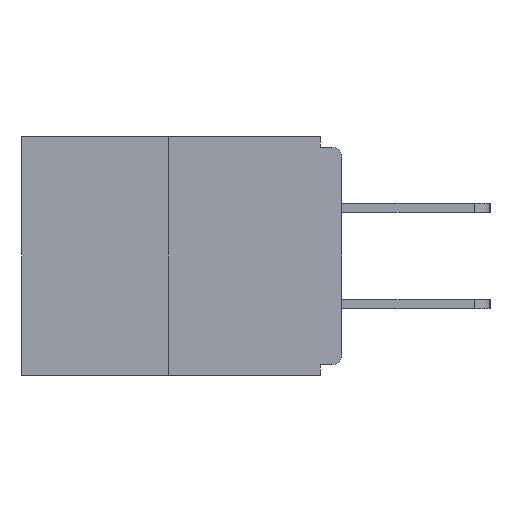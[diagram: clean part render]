
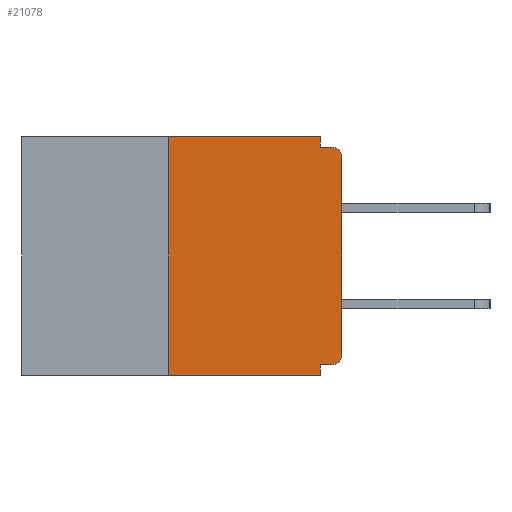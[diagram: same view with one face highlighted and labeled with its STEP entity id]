
A CAD part, left-side view. The second image highlights one B-rep face of the part: STEP entity #21078.
In plain terms, the highlighted planar face has unit normal (-1, 0, 0).
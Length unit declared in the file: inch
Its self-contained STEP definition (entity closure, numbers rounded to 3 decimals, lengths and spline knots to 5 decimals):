
#371 = CARTESIAN_POINT ( 'NONE',  ( 0., 0.031, 0. ) ) ;
#512 = EDGE_CURVE ( 'NONE', #14580, #19219, #6416, .T. ) ;
#513 = LINE ( 'NONE', #1695, #10660 ) ;
#1212 = ORIENTED_EDGE ( 'NONE', *, *, #22237, .T. ) ;
#1596 = DIRECTION ( 'NONE',  ( 0., 0., -1. ) ) ;
#1611 = VERTEX_POINT ( 'NONE', #3213 ) ;
#1613 = LINE ( 'NONE', #22744, #17285 ) ;
#1695 = CARTESIAN_POINT ( 'NONE',  ( 0., 0.031, -0.343 ) ) ;
#2230 = CARTESIAN_POINT ( 'NONE',  ( 0., 0.015, -0.03 ) ) ;
#3039 = VECTOR ( 'NONE', #11427, 39.37008 ) ;
#3213 = CARTESIAN_POINT ( 'NONE',  ( 0., 0., -0.03 ) ) ;
#3533 = PLANE ( 'NONE',  #20136 ) ;
#3790 = CARTESIAN_POINT ( 'NONE',  ( 0., 0.46, 0. ) ) ;
#3817 = VECTOR ( 'NONE', #20898, 39.37008 ) ;
#4071 = CARTESIAN_POINT ( 'NONE',  ( 0., 0., -0.313 ) ) ;
#4467 = LINE ( 'NONE', #14740, #19474 ) ;
#4643 = EDGE_CURVE ( 'NONE', #19219, #8950, #21563, .T. ) ;
#5315 = CARTESIAN_POINT ( 'NONE',  ( 0., 0.25, 0. ) ) ;
#5438 = LINE ( 'NONE', #5315, #3817 ) ;
#5472 = LINE ( 'NONE', #11512, #13109 ) ;
#6416 = LINE ( 'NONE', #6980, #3039 ) ;
#6980 = CARTESIAN_POINT ( 'NONE',  ( 0., 0.46, 0. ) ) ;
#7000 = CARTESIAN_POINT ( 'NONE',  ( 0., 0.031, -0.343 ) ) ;
#8950 = VERTEX_POINT ( 'NONE', #10053 ) ;
#8953 = EDGE_LOOP ( 'NONE', ( #13671, #9130, #1212, #21801, #15861, #16092, #9422, #15168, #15634, #17341 ) ) ;
#9130 = ORIENTED_EDGE ( 'NONE', *, *, #19822, .F. ) ;
#9142 = CARTESIAN_POINT ( 'NONE',  ( 0., 0.25, 0. ) ) ;
#9422 = ORIENTED_EDGE ( 'NONE', *, *, #11630, .T. ) ;
#9570 = DIRECTION ( 'NONE',  ( -1., 0., 0. ) ) ;
#9726 = DIRECTION ( 'NONE',  ( -1., 0., 0. ) ) ;
#10053 = CARTESIAN_POINT ( 'NONE',  ( 0., 0.031, -0.015 ) ) ;
#10634 = LINE ( 'NONE', #19244, #16167 ) ;
#10660 = VECTOR ( 'NONE', #13285, 39.37008 ) ;
#11008 = AXIS2_PLACEMENT_3D ( 'NONE', #23364, #9570, #11538 ) ;
#11126 = VECTOR ( 'NONE', #11910, 39.37008 ) ;
#11427 = DIRECTION ( 'NONE',  ( 0., -1., 0. ) ) ;
#11512 = CARTESIAN_POINT ( 'NONE',  ( 0., 0., -0.015 ) ) ;
#11538 = DIRECTION ( 'NONE',  ( 0., 0., -1. ) ) ;
#11630 = EDGE_CURVE ( 'NONE', #12138, #1611, #10634, .T. ) ;
#11910 = DIRECTION ( 'NONE',  ( 0., 0., -1. ) ) ;
#11997 = CARTESIAN_POINT ( 'NONE',  ( 0., 0.031, 0. ) ) ;
#12003 = VERTEX_POINT ( 'NONE', #25382 ) ;
#12138 = VERTEX_POINT ( 'NONE', #4071 ) ;
#12687 = VERTEX_POINT ( 'NONE', #7000 ) ;
#12958 = CARTESIAN_POINT ( 'NONE',  ( 0., 0.015, -0.015 ) ) ;
#13109 = VECTOR ( 'NONE', #21351, 39.37008 ) ;
#13216 = EDGE_CURVE ( 'NONE', #13564, #12003, #4467, .T. ) ;
#13285 = DIRECTION ( 'NONE',  ( 0., 0., -1. ) ) ;
#13564 = VERTEX_POINT ( 'NONE', #24943 ) ;
#13671 = ORIENTED_EDGE ( 'NONE', *, *, #512, .F. ) ;
#14247 = VERTEX_POINT ( 'NONE', #12958 ) ;
#14580 = VERTEX_POINT ( 'NONE', #9142 ) ;
#14707 = AXIS2_PLACEMENT_3D ( 'NONE', #2230, #9726, #15957 ) ;
#14740 = CARTESIAN_POINT ( 'NONE',  ( 0., 0., -0.328 ) ) ;
#15127 = EDGE_CURVE ( 'NONE', #1611, #14247, #25037, .T. ) ;
#15168 = ORIENTED_EDGE ( 'NONE', *, *, #15127, .T. ) ;
#15634 = ORIENTED_EDGE ( 'NONE', *, *, #19418, .F. ) ;
#15861 = ORIENTED_EDGE ( 'NONE', *, *, #13216, .F. ) ;
#15895 = VERTEX_POINT ( 'NONE', #23203 ) ;
#15957 = DIRECTION ( 'NONE',  ( 0., 0., -1. ) ) ;
#16092 = ORIENTED_EDGE ( 'NONE', *, *, #17820, .T. ) ;
#16167 = VECTOR ( 'NONE', #25067, 39.37008 ) ;
#17285 = VECTOR ( 'NONE', #22821, 39.37008 ) ;
#17341 = ORIENTED_EDGE ( 'NONE', *, *, #4643, .F. ) ;
#17820 = EDGE_CURVE ( 'NONE', #13564, #12138, #22434, .T. ) ;
#19219 = VERTEX_POINT ( 'NONE', #371 ) ;
#19244 = CARTESIAN_POINT ( 'NONE',  ( 0., 0., 0. ) ) ;
#19398 = EDGE_CURVE ( 'NONE', #12003, #12687, #513, .T. ) ;
#19418 = EDGE_CURVE ( 'NONE', #8950, #14247, #5472, .T. ) ;
#19474 = VECTOR ( 'NONE', #20687, 39.37008 ) ;
#19822 = EDGE_CURVE ( 'NONE', #15895, #14580, #5438, .T. ) ;
#20136 = AXIS2_PLACEMENT_3D ( 'NONE', #3790, #25098, #1596 ) ;
#20687 = DIRECTION ( 'NONE',  ( 0., 1., 0. ) ) ;
#20898 = DIRECTION ( 'NONE',  ( 0., 0., 1. ) ) ;
#21078 = ADVANCED_FACE ( 'NONE', ( #24409 ), #3533, .F. ) ;
#21351 = DIRECTION ( 'NONE',  ( 0., -1., 0. ) ) ;
#21563 = LINE ( 'NONE', #11997, #11126 ) ;
#21801 = ORIENTED_EDGE ( 'NONE', *, *, #19398, .F. ) ;
#22237 = EDGE_CURVE ( 'NONE', #15895, #12687, #1613, .T. ) ;
#22434 = CIRCLE ( 'NONE', #11008, 0.015 ) ;
#22744 = CARTESIAN_POINT ( 'NONE',  ( 0., 0.46, -0.343 ) ) ;
#22821 = DIRECTION ( 'NONE',  ( 0., -1., 0. ) ) ;
#23203 = CARTESIAN_POINT ( 'NONE',  ( 0., 0.25, -0.343 ) ) ;
#23364 = CARTESIAN_POINT ( 'NONE',  ( 0., 0.015, -0.313 ) ) ;
#24409 = FACE_OUTER_BOUND ( 'NONE', #8953, .T. ) ;
#24943 = CARTESIAN_POINT ( 'NONE',  ( 0., 0.015, -0.328 ) ) ;
#25037 = CIRCLE ( 'NONE', #14707, 0.015 ) ;
#25067 = DIRECTION ( 'NONE',  ( 0., 0., 1. ) ) ;
#25098 = DIRECTION ( 'NONE',  ( 1., 0., 0. ) ) ;
#25382 = CARTESIAN_POINT ( 'NONE',  ( 0., 0.031, -0.328 ) ) ;
